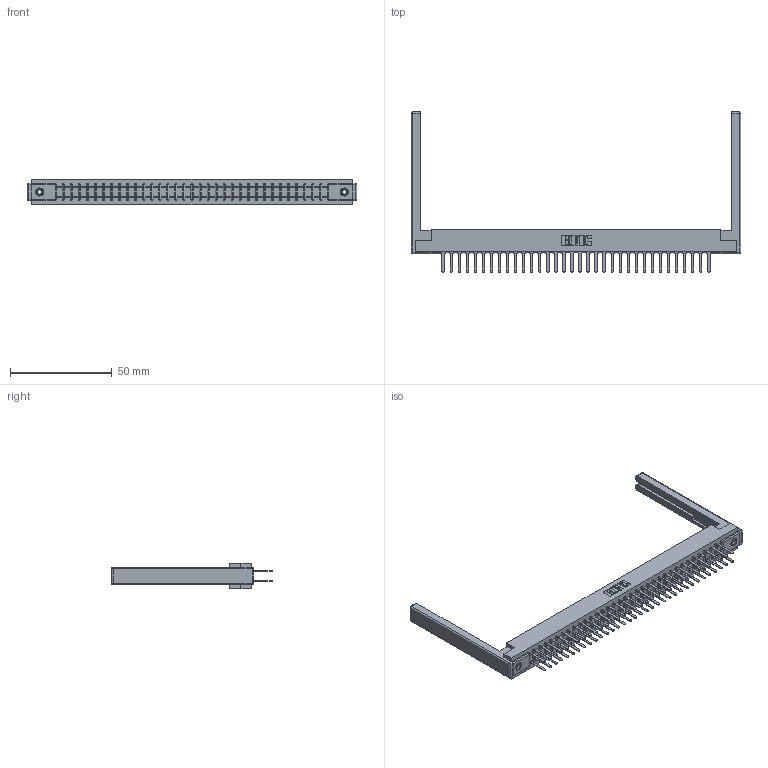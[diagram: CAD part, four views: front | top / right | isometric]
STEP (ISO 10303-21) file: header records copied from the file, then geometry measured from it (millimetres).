
FILE_DESCRIPTION (( 'STEP AP203' ), '1' );
FILE_NAME ('357-068-522-268.STEP', '2019-09-19T09:22:14', ( '' ), ( '' ), 'SwSTEP 2.0', 'SolidWorks 2016', '' );
FILE_SCHEMA (( 'CONFIG_CONTROL_DESIGN' ));
Length unit declared in the file: inch
Products named in the file (5): 345-250-001_345-250-001-102; 307-290-001_522; 307-220-068; 357-068-522-268; 307 Part_.156 Dia Mounting Holes
Assembly tree (73 placements, depth 2):
  357-068-522-268
    307 Part_.156 Dia Mounting Holes
    307-290-001_522  x68
    307-220-068  x2
    345-250-001_345-250-001-102  x2
Bounding box: 162.15 x 79.07 x 12.7 mm (x, y, z)
Volume: 21713.5 mm3; surface area: 25769.9 mm2
Topology: 73 solids, 73 shells, 3435 faces, 9553 edges, 6162 vertices
Faces by surface type: plane 2266, cylinder 1075, sphere 78, cone 12, torus 4
Entity records: 33949 total; most frequent: CARTESIAN_POINT 5531, ORIENTED_EDGE 5472, DIRECTION 5436, EDGE_CURVE 2736, LINE 2094, VECTOR 2094, VERTEX_POINT 1766, AXIS2_PLACEMENT_3D 1671
